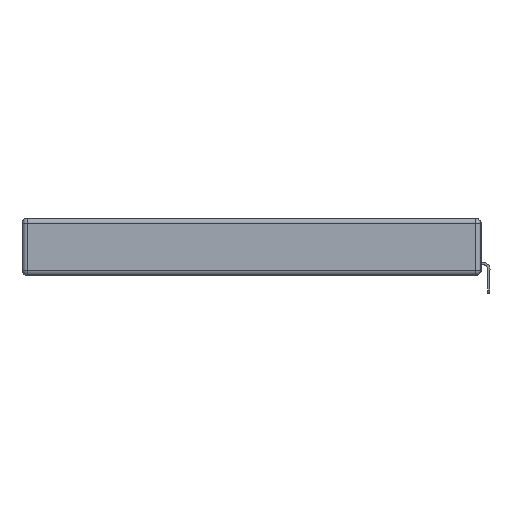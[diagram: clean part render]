
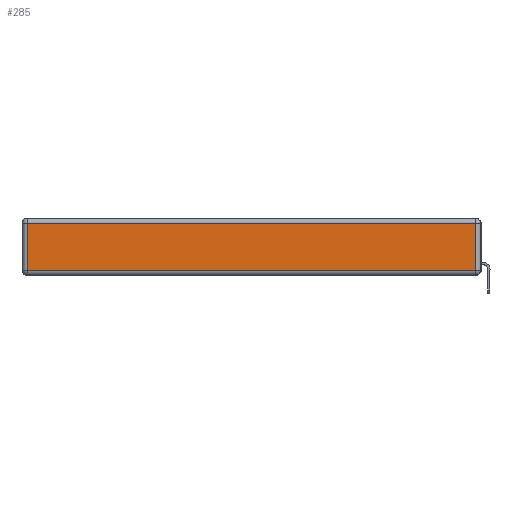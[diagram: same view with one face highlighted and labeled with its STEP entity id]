
A CAD part, left-side view. The second image highlights one B-rep face of the part: STEP entity #285.
In plain terms, the highlighted planar face has unit normal (-1, 0, 0).
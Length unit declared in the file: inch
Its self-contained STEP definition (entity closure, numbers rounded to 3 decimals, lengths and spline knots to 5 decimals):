
#285 = ADVANCED_FACE ( 'NONE', ( #28359 ), #22195, .T. ) ;
#776 = ORIENTED_EDGE ( 'NONE', *, *, #7128, .T. ) ;
#958 = LINE ( 'NONE', #12401, #9965 ) ;
#1440 = EDGE_CURVE ( 'NONE', #8322, #26141, #958, .T. ) ;
#1849 = DIRECTION ( 'NONE',  ( 0., -1., 0. ) ) ;
#2601 = LINE ( 'NONE', #3843, #3314 ) ;
#3314 = VECTOR ( 'NONE', #23663, 39.37008 ) ;
#3843 = CARTESIAN_POINT ( 'NONE',  ( 0., 2.72, -0.343 ) ) ;
#4305 = DIRECTION ( 'NONE',  ( -1., 0., 0. ) ) ;
#7128 = EDGE_CURVE ( 'NONE', #24412, #13587, #2601, .T. ) ;
#8322 = VERTEX_POINT ( 'NONE', #21277 ) ;
#9550 = CARTESIAN_POINT ( 'NONE',  ( 0., 2.72, -0.03 ) ) ;
#9965 = VECTOR ( 'NONE', #27658, 39.37008 ) ;
#10929 = DIRECTION ( 'NONE',  ( 0., 0., 1. ) ) ;
#11538 = CARTESIAN_POINT ( 'NONE',  ( 0., 2.72, -0.313 ) ) ;
#11586 = EDGE_CURVE ( 'NONE', #13587, #8322, #18220, .T. ) ;
#12401 = CARTESIAN_POINT ( 'NONE',  ( 0., 0.03, -0.343 ) ) ;
#13000 = CARTESIAN_POINT ( 'NONE',  ( 0., 2.75, -0.03 ) ) ;
#13587 = VERTEX_POINT ( 'NONE', #11538 ) ;
#13881 = VECTOR ( 'NONE', #26613, 39.37008 ) ;
#14112 = AXIS2_PLACEMENT_3D ( 'NONE', #24231, #4305, #10929 ) ;
#15133 = EDGE_CURVE ( 'NONE', #26141, #24412, #18041, .T. ) ;
#17490 = ORIENTED_EDGE ( 'NONE', *, *, #1440, .T. ) ;
#18041 = LINE ( 'NONE', #13000, #13881 ) ;
#18220 = LINE ( 'NONE', #19678, #23737 ) ;
#19678 = CARTESIAN_POINT ( 'NONE',  ( 0., 0., -0.313 ) ) ;
#20665 = ORIENTED_EDGE ( 'NONE', *, *, #11586, .T. ) ;
#21277 = CARTESIAN_POINT ( 'NONE',  ( 0., 0.03, -0.313 ) ) ;
#21703 = ORIENTED_EDGE ( 'NONE', *, *, #15133, .T. ) ;
#21937 = CARTESIAN_POINT ( 'NONE',  ( 0., 0.03, -0.03 ) ) ;
#22195 = PLANE ( 'NONE',  #14112 ) ;
#23663 = DIRECTION ( 'NONE',  ( 0., 0., -1. ) ) ;
#23737 = VECTOR ( 'NONE', #1849, 39.37008 ) ;
#24231 = CARTESIAN_POINT ( 'NONE',  ( 0., 0., -0.343 ) ) ;
#24412 = VERTEX_POINT ( 'NONE', #9550 ) ;
#26141 = VERTEX_POINT ( 'NONE', #21937 ) ;
#26613 = DIRECTION ( 'NONE',  ( 0., 1., 0. ) ) ;
#27658 = DIRECTION ( 'NONE',  ( 0., 0., 1. ) ) ;
#28359 = FACE_OUTER_BOUND ( 'NONE', #28430, .T. ) ;
#28430 = EDGE_LOOP ( 'NONE', ( #20665, #17490, #21703, #776 ) ) ;
